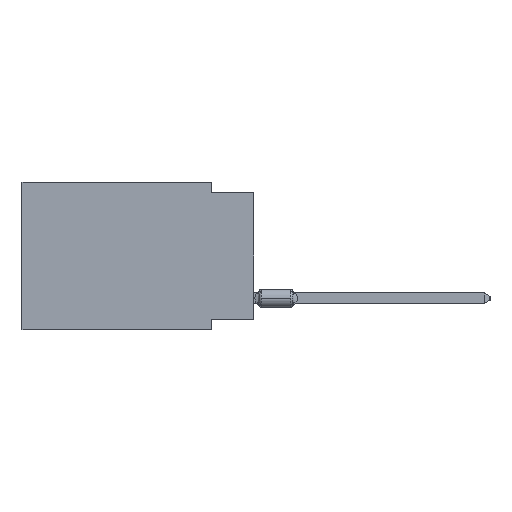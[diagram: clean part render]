
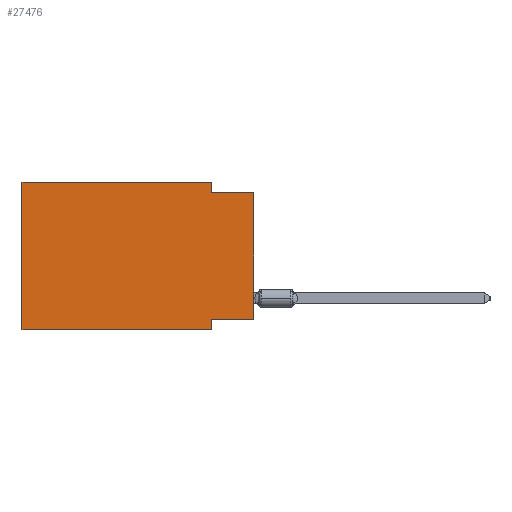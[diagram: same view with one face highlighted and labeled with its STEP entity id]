
A CAD part, left-side view. The second image highlights one B-rep face of the part: STEP entity #27476.
In plain terms, the highlighted planar face has unit normal (-1, 0, 0).
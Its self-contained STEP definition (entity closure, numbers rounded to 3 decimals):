
#1282 = VERTEX_POINT ( 'NONE', #50203 ) ;
#1761 = CARTESIAN_POINT ( 'NONE',  ( 0., 13.97, 0. ) ) ;
#2439 = EDGE_CURVE ( 'NONE', #37583, #25766, #21301, .T. ) ;
#4357 = DIRECTION ( 'NONE',  ( 1., 0., 0. ) ) ;
#4587 = ORIENTED_EDGE ( 'NONE', *, *, #2439, .F. ) ;
#5630 = CARTESIAN_POINT ( 'NONE',  ( 0., 13.97, 0. ) ) ;
#6417 = LINE ( 'NONE', #51784, #55280 ) ;
#9077 = CARTESIAN_POINT ( 'NONE',  ( 0., 13.97, 0. ) ) ;
#9322 = EDGE_CURVE ( 'NONE', #50221, #1282, #30596, .T. ) ;
#10254 = CARTESIAN_POINT ( 'NONE',  ( 0., 2.54, 0. ) ) ;
#10517 = EDGE_CURVE ( 'NONE', #38937, #1282, #45032, .T. ) ;
#14097 = CARTESIAN_POINT ( 'NONE',  ( 0., 2.54, -0.635 ) ) ;
#14267 = CARTESIAN_POINT ( 'NONE',  ( 0., 0., 0. ) ) ;
#15863 = EDGE_CURVE ( 'NONE', #22020, #48756, #51068, .T. ) ;
#17526 = VECTOR ( 'NONE', #53863, 1000. ) ;
#18172 = LINE ( 'NONE', #9077, #35771 ) ;
#21301 = LINE ( 'NONE', #39602, #27769 ) ;
#22020 = VERTEX_POINT ( 'NONE', #45971 ) ;
#22218 = AXIS2_PLACEMENT_3D ( 'NONE', #29987, #4357, #22292 ) ;
#22292 = DIRECTION ( 'NONE',  ( 0., 0., -1. ) ) ;
#23452 = DIRECTION ( 'NONE',  ( 0., 1., 0. ) ) ;
#23540 = DIRECTION ( 'NONE',  ( 0., 0., 1. ) ) ;
#25766 = VERTEX_POINT ( 'NONE', #14097 ) ;
#26449 = DIRECTION ( 'NONE',  ( 0., -1., 0. ) ) ;
#26455 = VECTOR ( 'NONE', #26449, 1000. ) ;
#26708 = PLANE ( 'NONE',  #22218 ) ;
#27476 = ADVANCED_FACE ( 'NONE', ( #49181 ), #26708, .F. ) ;
#27524 = DIRECTION ( 'NONE',  ( 0., 0., 1. ) ) ;
#27769 = VECTOR ( 'NONE', #49349, 1000. ) ;
#28390 = CARTESIAN_POINT ( 'NONE',  ( 0., 0., -0.635 ) ) ;
#29987 = CARTESIAN_POINT ( 'NONE',  ( 0., 13.97, 0. ) ) ;
#30596 = LINE ( 'NONE', #36196, #26455 ) ;
#31288 = CARTESIAN_POINT ( 'NONE',  ( 0., 13.97, -8.89 ) ) ;
#32012 = LINE ( 'NONE', #50042, #44506 ) ;
#32066 = EDGE_CURVE ( 'NONE', #22020, #38937, #6417, .T. ) ;
#32605 = DIRECTION ( 'NONE',  ( 0., -1., 0. ) ) ;
#33370 = ORIENTED_EDGE ( 'NONE', *, *, #32066, .F. ) ;
#34050 = ORIENTED_EDGE ( 'NONE', *, *, #48053, .F. ) ;
#34274 = ORIENTED_EDGE ( 'NONE', *, *, #10517, .F. ) ;
#35771 = VECTOR ( 'NONE', #40603, 1000. ) ;
#35870 = CARTESIAN_POINT ( 'NONE',  ( 0., 2.54, -8.89 ) ) ;
#36196 = CARTESIAN_POINT ( 'NONE',  ( 0., 13.97, -8.89 ) ) ;
#36342 = VECTOR ( 'NONE', #23540, 1000. ) ;
#37583 = VERTEX_POINT ( 'NONE', #10254 ) ;
#38507 = EDGE_CURVE ( 'NONE', #50221, #46889, #46005, .T. ) ;
#38893 = VECTOR ( 'NONE', #27524, 1000. ) ;
#38937 = VERTEX_POINT ( 'NONE', #47082 ) ;
#39602 = CARTESIAN_POINT ( 'NONE',  ( 0., 2.54, 0. ) ) ;
#40603 = DIRECTION ( 'NONE',  ( 0., -1., 0. ) ) ;
#42288 = EDGE_CURVE ( 'NONE', #46889, #37583, #18172, .T. ) ;
#42353 = ORIENTED_EDGE ( 'NONE', *, *, #38507, .F. ) ;
#44506 = VECTOR ( 'NONE', #32605, 1000. ) ;
#44616 = EDGE_LOOP ( 'NONE', ( #54607, #34050, #4587, #51252, #42353, #57957, #34274, #33370 ) ) ;
#45032 = LINE ( 'NONE', #35870, #17526 ) ;
#45971 = CARTESIAN_POINT ( 'NONE',  ( 0., 0., -8.255 ) ) ;
#46005 = LINE ( 'NONE', #5630, #36342 ) ;
#46889 = VERTEX_POINT ( 'NONE', #1761 ) ;
#47082 = CARTESIAN_POINT ( 'NONE',  ( 0., 2.54, -8.255 ) ) ;
#48053 = EDGE_CURVE ( 'NONE', #25766, #48756, #32012, .T. ) ;
#48756 = VERTEX_POINT ( 'NONE', #28390 ) ;
#49181 = FACE_OUTER_BOUND ( 'NONE', #44616, .T. ) ;
#49349 = DIRECTION ( 'NONE',  ( 0., 0., -1. ) ) ;
#50042 = CARTESIAN_POINT ( 'NONE',  ( 0., 0., -0.635 ) ) ;
#50203 = CARTESIAN_POINT ( 'NONE',  ( 0., 2.54, -8.89 ) ) ;
#50221 = VERTEX_POINT ( 'NONE', #31288 ) ;
#51068 = LINE ( 'NONE', #14267, #38893 ) ;
#51252 = ORIENTED_EDGE ( 'NONE', *, *, #42288, .F. ) ;
#51784 = CARTESIAN_POINT ( 'NONE',  ( 0., 0., -8.255 ) ) ;
#53863 = DIRECTION ( 'NONE',  ( 0., 0., -1. ) ) ;
#54607 = ORIENTED_EDGE ( 'NONE', *, *, #15863, .T. ) ;
#55280 = VECTOR ( 'NONE', #23452, 1000. ) ;
#57957 = ORIENTED_EDGE ( 'NONE', *, *, #9322, .T. ) ;
